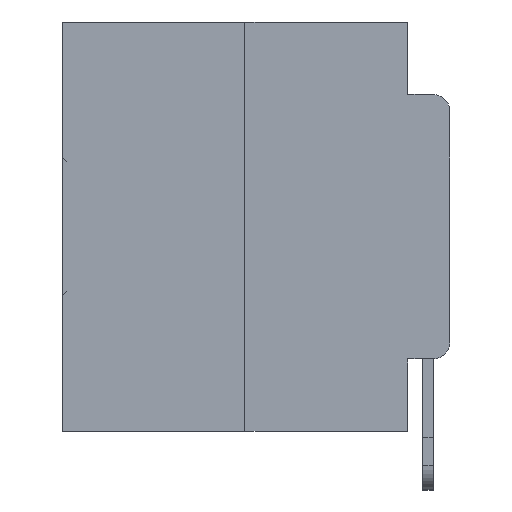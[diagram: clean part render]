
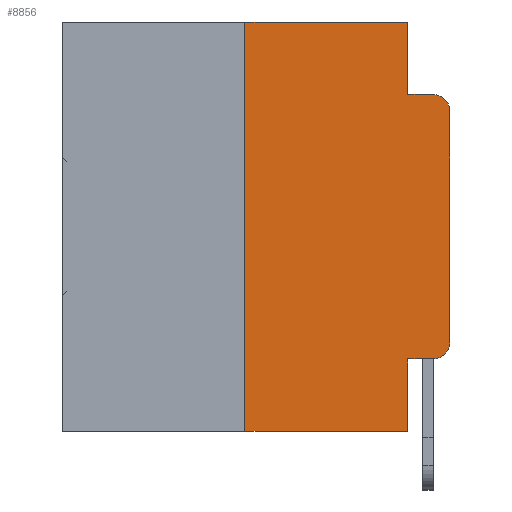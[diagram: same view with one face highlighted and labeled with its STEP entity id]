
A CAD part, left-side view. The second image highlights one B-rep face of the part: STEP entity #8856.
In plain terms, the highlighted planar face has unit normal (-1, 0, 0).
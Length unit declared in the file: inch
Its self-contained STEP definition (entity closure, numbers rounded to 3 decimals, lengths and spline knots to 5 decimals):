
#422 = CARTESIAN_POINT ( 'NONE',  ( 0., 0.051, 0. ) ) ;
#888 = ORIENTED_EDGE ( 'NONE', *, *, #21455, .T. ) ;
#1006 = ORIENTED_EDGE ( 'NONE', *, *, #11407, .T. ) ;
#3041 = EDGE_CURVE ( 'NONE', #23053, #12543, #4312, .T. ) ;
#3100 = LINE ( 'NONE', #8850, #28378 ) ;
#3116 = PLANE ( 'NONE',  #21056 ) ;
#4243 = CARTESIAN_POINT ( 'NONE',  ( 0., 0.02, -0.4115 ) ) ;
#4312 = LINE ( 'NONE', #12688, #10472 ) ;
#4360 = LINE ( 'NONE', #29759, #16531 ) ;
#4884 = DIRECTION ( 'NONE',  ( 0., 0., -1. ) ) ;
#4934 = ORIENTED_EDGE ( 'NONE', *, *, #29489, .T. ) ;
#5759 = CIRCLE ( 'NONE', #20327, 0.02 ) ;
#5809 = DIRECTION ( 'NONE',  ( 0., 0., -1. ) ) ;
#7240 = EDGE_LOOP ( 'NONE', ( #1006, #888, #18769, #8020, #30814, #24479, #9421, #16295, #21789, #4934 ) ) ;
#7763 = LINE ( 'NONE', #26876, #21200 ) ;
#8020 = ORIENTED_EDGE ( 'NONE', *, *, #20844, .F. ) ;
#8236 = VECTOR ( 'NONE', #23525, 39.37008 ) ;
#8264 = CARTESIAN_POINT ( 'NONE',  ( 0., 0., 0. ) ) ;
#8483 = EDGE_CURVE ( 'NONE', #15294, #12543, #7763, .T. ) ;
#8500 = VERTEX_POINT ( 'NONE', #24440 ) ;
#8850 = CARTESIAN_POINT ( 'NONE',  ( 0., 0.473, 0. ) ) ;
#8856 = ADVANCED_FACE ( 'NONE', ( #20419 ), #3116, .F. ) ;
#9303 = CARTESIAN_POINT ( 'NONE',  ( 0., 0.051, -0.5 ) ) ;
#9421 = ORIENTED_EDGE ( 'NONE', *, *, #8483, .T. ) ;
#9575 = CARTESIAN_POINT ( 'NONE',  ( 0., 0.25, 0. ) ) ;
#9864 = CARTESIAN_POINT ( 'NONE',  ( 0., 0.02, -0.1085 ) ) ;
#10472 = VECTOR ( 'NONE', #4884, 39.37008 ) ;
#11407 = EDGE_CURVE ( 'NONE', #12231, #20001, #24116, .T. ) ;
#12064 = DIRECTION ( 'NONE',  ( 0., -1., 0. ) ) ;
#12231 = VERTEX_POINT ( 'NONE', #22728 ) ;
#12518 = DIRECTION ( 'NONE',  ( 0., 0., -1. ) ) ;
#12543 = VERTEX_POINT ( 'NONE', #9303 ) ;
#12688 = CARTESIAN_POINT ( 'NONE',  ( 0., 0.051, 0. ) ) ;
#13591 = CARTESIAN_POINT ( 'NONE',  ( 0., 0.051, 0. ) ) ;
#14253 = CARTESIAN_POINT ( 'NONE',  ( 0., 0.02, -0.3915 ) ) ;
#14708 = DIRECTION ( 'NONE',  ( 0., -1., 0. ) ) ;
#15294 = VERTEX_POINT ( 'NONE', #24010 ) ;
#15434 = VECTOR ( 'NONE', #27363, 39.37008 ) ;
#15513 = AXIS2_PLACEMENT_3D ( 'NONE', #14253, #31385, #16764 ) ;
#16000 = CIRCLE ( 'NONE', #15513, 0.02 ) ;
#16295 = ORIENTED_EDGE ( 'NONE', *, *, #3041, .F. ) ;
#16359 = EDGE_CURVE ( 'NONE', #29639, #32460, #3100, .T. ) ;
#16531 = VECTOR ( 'NONE', #32195, 39.37008 ) ;
#16764 = DIRECTION ( 'NONE',  ( 0., 0., -1. ) ) ;
#17637 = VECTOR ( 'NONE', #18848, 39.37008 ) ;
#18087 = CARTESIAN_POINT ( 'NONE',  ( 0., 0.051, -0.0885 ) ) ;
#18239 = CARTESIAN_POINT ( 'NONE',  ( 0., 0., -0.1085 ) ) ;
#18769 = ORIENTED_EDGE ( 'NONE', *, *, #23086, .F. ) ;
#18848 = DIRECTION ( 'NONE',  ( 0., 0., 1. ) ) ;
#19653 = EDGE_CURVE ( 'NONE', #23053, #28208, #28505, .T. ) ;
#20001 = VERTEX_POINT ( 'NONE', #18239 ) ;
#20327 = AXIS2_PLACEMENT_3D ( 'NONE', #9864, #27287, #12518 ) ;
#20419 = FACE_OUTER_BOUND ( 'NONE', #7240, .T. ) ;
#20844 = EDGE_CURVE ( 'NONE', #32460, #31791, #22437, .T. ) ;
#21026 = DIRECTION ( 'NONE',  ( 1., 0., 0. ) ) ;
#21056 = AXIS2_PLACEMENT_3D ( 'NONE', #28290, #21026, #5809 ) ;
#21200 = VECTOR ( 'NONE', #12064, 39.37008 ) ;
#21242 = VECTOR ( 'NONE', #14708, 39.37008 ) ;
#21455 = EDGE_CURVE ( 'NONE', #20001, #8500, #5759, .T. ) ;
#21789 = ORIENTED_EDGE ( 'NONE', *, *, #19653, .T. ) ;
#21898 = CARTESIAN_POINT ( 'NONE',  ( 0., 0.051, -0.4115 ) ) ;
#22091 = CARTESIAN_POINT ( 'NONE',  ( 0., 0.051, -0.4115 ) ) ;
#22437 = LINE ( 'NONE', #422, #8236 ) ;
#22446 = CARTESIAN_POINT ( 'NONE',  ( 0., 0.051, -0.0885 ) ) ;
#22728 = CARTESIAN_POINT ( 'NONE',  ( 0., 0., -0.3915 ) ) ;
#23053 = VERTEX_POINT ( 'NONE', #21898 ) ;
#23086 = EDGE_CURVE ( 'NONE', #31791, #8500, #29183, .T. ) ;
#23525 = DIRECTION ( 'NONE',  ( 0., 0., -1. ) ) ;
#24010 = CARTESIAN_POINT ( 'NONE',  ( 0., 0.25, -0.5 ) ) ;
#24116 = LINE ( 'NONE', #8264, #17637 ) ;
#24440 = CARTESIAN_POINT ( 'NONE',  ( 0., 0.02, -0.0885 ) ) ;
#24479 = ORIENTED_EDGE ( 'NONE', *, *, #27406, .F. ) ;
#26876 = CARTESIAN_POINT ( 'NONE',  ( 0., 0.473, -0.5 ) ) ;
#27287 = DIRECTION ( 'NONE',  ( -1., 0., 0. ) ) ;
#27363 = DIRECTION ( 'NONE',  ( 0., -1., 0. ) ) ;
#27406 = EDGE_CURVE ( 'NONE', #15294, #29639, #4360, .T. ) ;
#28208 = VERTEX_POINT ( 'NONE', #4243 ) ;
#28290 = CARTESIAN_POINT ( 'NONE',  ( 0., 0.473, 0. ) ) ;
#28378 = VECTOR ( 'NONE', #31253, 39.37008 ) ;
#28505 = LINE ( 'NONE', #22091, #21242 ) ;
#29183 = LINE ( 'NONE', #22446, #15434 ) ;
#29489 = EDGE_CURVE ( 'NONE', #28208, #12231, #16000, .T. ) ;
#29639 = VERTEX_POINT ( 'NONE', #9575 ) ;
#29759 = CARTESIAN_POINT ( 'NONE',  ( 0., 0.25, 0. ) ) ;
#30814 = ORIENTED_EDGE ( 'NONE', *, *, #16359, .F. ) ;
#31253 = DIRECTION ( 'NONE',  ( 0., -1., 0. ) ) ;
#31385 = DIRECTION ( 'NONE',  ( -1., 0., 0. ) ) ;
#31791 = VERTEX_POINT ( 'NONE', #18087 ) ;
#32195 = DIRECTION ( 'NONE',  ( 0., 0., 1. ) ) ;
#32460 = VERTEX_POINT ( 'NONE', #13591 ) ;
